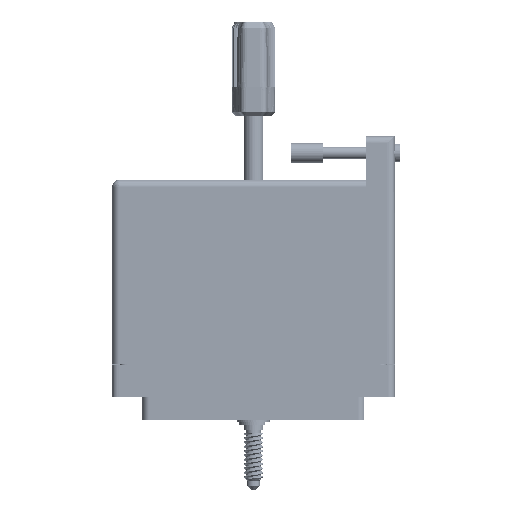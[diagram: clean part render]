
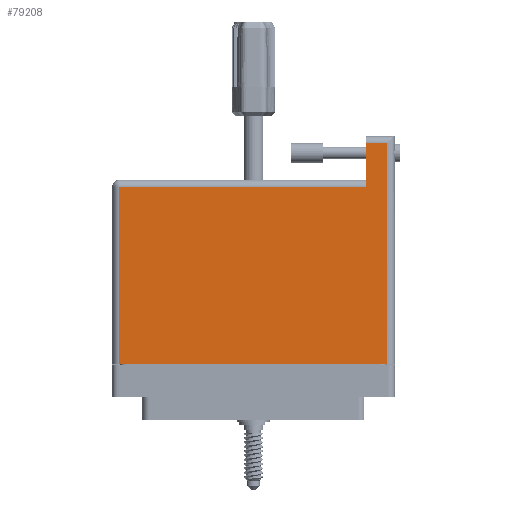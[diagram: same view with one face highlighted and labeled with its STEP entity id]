
A CAD part, front view. The second image highlights one B-rep face of the part: STEP entity #79208.
In plain terms, the highlighted face is planar.
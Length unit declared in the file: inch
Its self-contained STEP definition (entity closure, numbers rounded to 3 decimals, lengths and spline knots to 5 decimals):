
#3463 = DIRECTION ( 'NONE',  ( -1., 0., 0. ) ) ;
#7105 = LINE ( 'NONE', #34573, #34316 ) ;
#12068 = CARTESIAN_POINT ( 'NONE',  ( 1.079, 2.095, 0.617 ) ) ;
#12956 = EDGE_CURVE ( 'NONE', #49790, #31023, #33859, .T. ) ;
#13051 = CARTESIAN_POINT ( 'NONE',  ( 1.079, 1.605, 0.617 ) ) ;
#15574 = CARTESIAN_POINT ( 'NONE',  ( -1.359, 1.605, 0.617 ) ) ;
#15939 = ORIENTED_EDGE ( 'NONE', *, *, #12956, .T. ) ;
#16062 = VECTOR ( 'NONE', #26121, 39.37008 ) ;
#17791 = CARTESIAN_POINT ( 'NONE',  ( -1.359, 2.025, 0.617 ) ) ;
#19890 = CARTESIAN_POINT ( 'NONE',  ( -1.289, -0.1, 0.617 ) ) ;
#21234 = CARTESIAN_POINT ( 'NONE',  ( -1.359, 1.675, 0.617 ) ) ;
#21841 = DIRECTION ( 'NONE',  ( 1., 0., 0. ) ) ;
#22245 = LINE ( 'NONE', #15574, #55815 ) ;
#23393 = VERTEX_POINT ( 'NONE', #84265 ) ;
#24152 = VECTOR ( 'NONE', #3463, 39.37008 ) ;
#26121 = DIRECTION ( 'NONE',  ( 0., -1., 0. ) ) ;
#28540 = EDGE_CURVE ( 'NONE', #32760, #23393, #39345, .T. ) ;
#31023 = VERTEX_POINT ( 'NONE', #13051 ) ;
#32760 = VERTEX_POINT ( 'NONE', #46850 ) ;
#33859 = LINE ( 'NONE', #12068, #16062 ) ;
#34110 = VECTOR ( 'NONE', #21841, 39.37008 ) ;
#34314 = FACE_OUTER_BOUND ( 'NONE', #67324, .T. ) ;
#34316 = VECTOR ( 'NONE', #41325, 39.37008 ) ;
#34573 = CARTESIAN_POINT ( 'NONE',  ( 1.289, 2.095, 0.617 ) ) ;
#36018 = EDGE_CURVE ( 'NONE', #79282, #49790, #44081, .T. ) ;
#39345 = LINE ( 'NONE', #42357, #34110 ) ;
#40798 = ORIENTED_EDGE ( 'NONE', *, *, #84228, .T. ) ;
#41325 = DIRECTION ( 'NONE',  ( 0., 1., 0. ) ) ;
#42357 = CARTESIAN_POINT ( 'NONE',  ( -1.359, -0.1, 0.617 ) ) ;
#44081 = LINE ( 'NONE', #17791, #24152 ) ;
#44199 = ORIENTED_EDGE ( 'NONE', *, *, #28540, .T. ) ;
#44823 = ORIENTED_EDGE ( 'NONE', *, *, #68121, .T. ) ;
#46850 = CARTESIAN_POINT ( 'NONE',  ( -1.289, -0.1, 0.617 ) ) ;
#48130 = DIRECTION ( 'NONE',  ( 0., 0., -1. ) ) ;
#49790 = VERTEX_POINT ( 'NONE', #60344 ) ;
#55815 = VECTOR ( 'NONE', #81640, 39.37008 ) ;
#56115 = DIRECTION ( 'NONE',  ( 0., -1., 0. ) ) ;
#56906 = ORIENTED_EDGE ( 'NONE', *, *, #63194, .T. ) ;
#57985 = ORIENTED_EDGE ( 'NONE', *, *, #36018, .T. ) ;
#60344 = CARTESIAN_POINT ( 'NONE',  ( 1.079, 2.025, 0.617 ) ) ;
#63194 = EDGE_CURVE ( 'NONE', #23393, #79282, #7105, .T. ) ;
#67324 = EDGE_LOOP ( 'NONE', ( #40798, #44823, #44199, #56906, #57985, #15939 ) ) ;
#67561 = CARTESIAN_POINT ( 'NONE',  ( -1.289, 1.605, 0.617 ) ) ;
#68121 = EDGE_CURVE ( 'NONE', #79777, #32760, #82387, .T. ) ;
#69410 = CARTESIAN_POINT ( 'NONE',  ( 1.289, 2.025, 0.617 ) ) ;
#74708 = DIRECTION ( 'NONE',  ( -1., 0., 0. ) ) ;
#76115 = VECTOR ( 'NONE', #56115, 39.37008 ) ;
#79208 = ADVANCED_FACE ( 'NONE', ( #34314 ), #81994, .F. ) ;
#79282 = VERTEX_POINT ( 'NONE', #69410 ) ;
#79777 = VERTEX_POINT ( 'NONE', #67561 ) ;
#81640 = DIRECTION ( 'NONE',  ( -1., 0., 0. ) ) ;
#81994 = PLANE ( 'NONE',  #84823 ) ;
#82387 = LINE ( 'NONE', #19890, #76115 ) ;
#84228 = EDGE_CURVE ( 'NONE', #31023, #79777, #22245, .T. ) ;
#84265 = CARTESIAN_POINT ( 'NONE',  ( 1.289, -0.1, 0.617 ) ) ;
#84823 = AXIS2_PLACEMENT_3D ( 'NONE', #21234, #48130, #74708 ) ;
